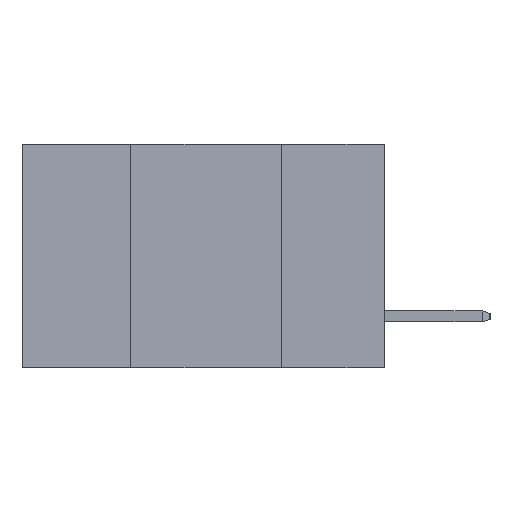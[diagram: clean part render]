
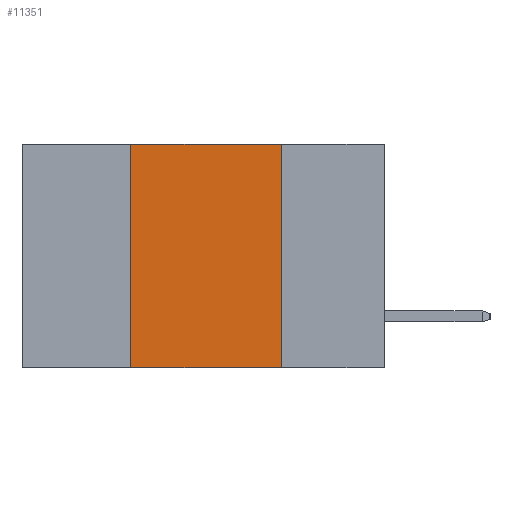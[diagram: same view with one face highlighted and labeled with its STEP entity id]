
A CAD part, left-side view. The second image highlights one B-rep face of the part: STEP entity #11351.
In plain terms, the highlighted planar face has unit normal (-1, 0, 0).
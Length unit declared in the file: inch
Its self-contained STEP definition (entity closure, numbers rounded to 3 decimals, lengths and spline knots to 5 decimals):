
#557 = CARTESIAN_POINT ( 'NONE',  ( 0., 0.6, -0.37 ) ) ;
#1002 = VERTEX_POINT ( 'NONE', #16184 ) ;
#1009 = VECTOR ( 'NONE', #12901, 39.37008 ) ;
#1423 = VECTOR ( 'NONE', #9341, 39.37008 ) ;
#2564 = DIRECTION ( 'NONE',  ( 0., 0., -1. ) ) ;
#3354 = CARTESIAN_POINT ( 'NONE',  ( 0., 0.42, 0. ) ) ;
#4069 = EDGE_CURVE ( 'NONE', #9070, #1002, #11649, .T. ) ;
#4315 = CARTESIAN_POINT ( 'NONE',  ( 0., 0.17, 0. ) ) ;
#4676 = CARTESIAN_POINT ( 'NONE',  ( 0., 0.42, -0.37 ) ) ;
#4771 = VECTOR ( 'NONE', #19349, 39.37008 ) ;
#7241 = CARTESIAN_POINT ( 'NONE',  ( 0., 0.42, 0. ) ) ;
#7527 = ORIENTED_EDGE ( 'NONE', *, *, #4069, .F. ) ;
#7729 = CARTESIAN_POINT ( 'NONE',  ( 0., 0.6, 0. ) ) ;
#9070 = VERTEX_POINT ( 'NONE', #16802 ) ;
#9341 = DIRECTION ( 'NONE',  ( 0., 0., 1. ) ) ;
#9818 = DIRECTION ( 'NONE',  ( 0., 0., -1. ) ) ;
#11227 = CARTESIAN_POINT ( 'NONE',  ( 0., 0.6, 0. ) ) ;
#11351 = ADVANCED_FACE ( 'NONE', ( #20254 ), #13812, .F. ) ;
#11649 = LINE ( 'NONE', #4315, #16437 ) ;
#11727 = ORIENTED_EDGE ( 'NONE', *, *, #23730, .F. ) ;
#12381 = LINE ( 'NONE', #7241, #1423 ) ;
#12621 = LINE ( 'NONE', #557, #1009 ) ;
#12901 = DIRECTION ( 'NONE',  ( 0., -1., 0. ) ) ;
#13217 = ORIENTED_EDGE ( 'NONE', *, *, #13271, .F. ) ;
#13271 = EDGE_CURVE ( 'NONE', #17936, #9070, #20451, .T. ) ;
#13812 = PLANE ( 'NONE',  #19509 ) ;
#16118 = EDGE_CURVE ( 'NONE', #23070, #1002, #12621, .T. ) ;
#16184 = CARTESIAN_POINT ( 'NONE',  ( 0., 0.17, -0.37 ) ) ;
#16437 = VECTOR ( 'NONE', #2564, 39.37008 ) ;
#16802 = CARTESIAN_POINT ( 'NONE',  ( 0., 0.17, 0. ) ) ;
#17671 = ORIENTED_EDGE ( 'NONE', *, *, #16118, .T. ) ;
#17936 = VERTEX_POINT ( 'NONE', #3354 ) ;
#19349 = DIRECTION ( 'NONE',  ( 0., -1., 0. ) ) ;
#19509 = AXIS2_PLACEMENT_3D ( 'NONE', #7729, #22023, #9818 ) ;
#20254 = FACE_OUTER_BOUND ( 'NONE', #26155, .T. ) ;
#20451 = LINE ( 'NONE', #11227, #4771 ) ;
#22023 = DIRECTION ( 'NONE',  ( 1., 0., 0. ) ) ;
#23070 = VERTEX_POINT ( 'NONE', #4676 ) ;
#23730 = EDGE_CURVE ( 'NONE', #23070, #17936, #12381, .T. ) ;
#26155 = EDGE_LOOP ( 'NONE', ( #7527, #13217, #11727, #17671 ) ) ;
